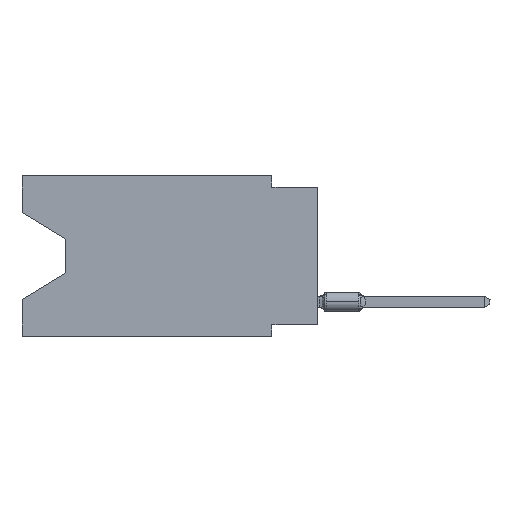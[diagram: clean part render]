
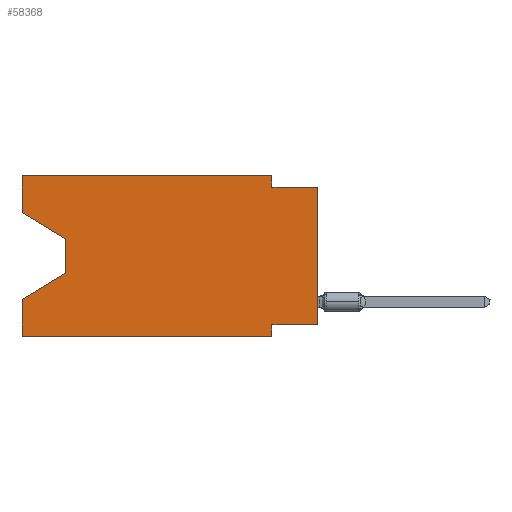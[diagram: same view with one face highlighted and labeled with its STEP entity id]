
A CAD part, left-side view. The second image highlights one B-rep face of the part: STEP entity #58368.
In plain terms, the highlighted planar face has unit normal (-1, 0, 0).
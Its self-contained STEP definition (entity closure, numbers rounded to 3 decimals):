
#1597 = DIRECTION ( 'NONE',  ( 0., -1., 0. ) ) ;
#2646 = CARTESIAN_POINT ( 'NONE',  ( 0., 16.383, -2.038 ) ) ;
#3016 = LINE ( 'NONE', #53191, #84202 ) ;
#3554 = LINE ( 'NONE', #24360, #45992 ) ;
#4073 = LINE ( 'NONE', #61832, #77702 ) ;
#5018 = DIRECTION ( 'NONE',  ( 0., 0., -1. ) ) ;
#6197 = VECTOR ( 'NONE', #53767, 1000. ) ;
#7446 = EDGE_CURVE ( 'NONE', #9179, #8577, #59473, .T. ) ;
#8342 = CARTESIAN_POINT ( 'NONE',  ( 0., 2.54, 0. ) ) ;
#8478 = CARTESIAN_POINT ( 'NONE',  ( 0., 16.383, 0. ) ) ;
#8577 = VERTEX_POINT ( 'NONE', #38698 ) ;
#9179 = VERTEX_POINT ( 'NONE', #23064 ) ;
#10538 = CARTESIAN_POINT ( 'NONE',  ( 0., 16.383, -6.852 ) ) ;
#14163 = ORIENTED_EDGE ( 'NONE', *, *, #7446, .F. ) ;
#16252 = CARTESIAN_POINT ( 'NONE',  ( 0., 0., -0.635 ) ) ;
#16510 = LINE ( 'NONE', #33056, #33289 ) ;
#17475 = CARTESIAN_POINT ( 'NONE',  ( 0., 13.97, -3.505 ) ) ;
#18274 = CARTESIAN_POINT ( 'NONE',  ( 0., 2.54, -8.89 ) ) ;
#18910 = ORIENTED_EDGE ( 'NONE', *, *, #53152, .F. ) ;
#22202 = LINE ( 'NONE', #8478, #68159 ) ;
#22275 = VERTEX_POINT ( 'NONE', #86862 ) ;
#23064 = CARTESIAN_POINT ( 'NONE',  ( 0., 2.54, 0. ) ) ;
#23119 = VERTEX_POINT ( 'NONE', #49735 ) ;
#23192 = CARTESIAN_POINT ( 'NONE',  ( 0., 16.383, 0. ) ) ;
#24360 = CARTESIAN_POINT ( 'NONE',  ( 0., 16.383, -8.89 ) ) ;
#24616 = ORIENTED_EDGE ( 'NONE', *, *, #71028, .T. ) ;
#26470 = EDGE_CURVE ( 'NONE', #22275, #47350, #39522, .T. ) ;
#27247 = LINE ( 'NONE', #18274, #87686 ) ;
#27259 = DIRECTION ( 'NONE',  ( 0., 0., 1. ) ) ;
#27795 = ORIENTED_EDGE ( 'NONE', *, *, #49248, .T. ) ;
#29065 = AXIS2_PLACEMENT_3D ( 'NONE', #48102, #54296, #53832 ) ;
#30268 = DIRECTION ( 'NONE',  ( 0., 0., 1. ) ) ;
#31049 = VECTOR ( 'NONE', #37221, 1000. ) ;
#31284 = VECTOR ( 'NONE', #34938, 1000. ) ;
#33056 = CARTESIAN_POINT ( 'NONE',  ( 0., 0., -8.255 ) ) ;
#33289 = VECTOR ( 'NONE', #83257, 1000. ) ;
#34938 = DIRECTION ( 'NONE',  ( 0., 0., -1. ) ) ;
#35866 = LINE ( 'NONE', #63342, #31284 ) ;
#37221 = DIRECTION ( 'NONE',  ( 0., 0., -1. ) ) ;
#38698 = CARTESIAN_POINT ( 'NONE',  ( 0., 2.54, -0.635 ) ) ;
#39522 = LINE ( 'NONE', #89206, #59727 ) ;
#42939 = VERTEX_POINT ( 'NONE', #63623 ) ;
#43797 = EDGE_CURVE ( 'NONE', #84030, #50709, #67022, .T. ) ;
#43973 = ORIENTED_EDGE ( 'NONE', *, *, #76779, .F. ) ;
#44457 = ORIENTED_EDGE ( 'NONE', *, *, #43797, .T. ) ;
#45992 = VECTOR ( 'NONE', #53250, 1000. ) ;
#47350 = VERTEX_POINT ( 'NONE', #10538 ) ;
#47457 = CARTESIAN_POINT ( 'NONE',  ( 0., 2.54, -8.255 ) ) ;
#48102 = CARTESIAN_POINT ( 'NONE',  ( 0., 16.383, 0. ) ) ;
#48496 = ORIENTED_EDGE ( 'NONE', *, *, #26470, .T. ) ;
#48751 = ORIENTED_EDGE ( 'NONE', *, *, #84985, .F. ) ;
#49248 = EDGE_CURVE ( 'NONE', #23119, #42939, #3554, .T. ) ;
#49735 = CARTESIAN_POINT ( 'NONE',  ( 0., 16.383, -8.89 ) ) ;
#50709 = VERTEX_POINT ( 'NONE', #17475 ) ;
#52830 = ORIENTED_EDGE ( 'NONE', *, *, #90267, .F. ) ;
#53152 = EDGE_CURVE ( 'NONE', #23119, #47350, #88065, .T. ) ;
#53191 = CARTESIAN_POINT ( 'NONE',  ( 0., 0., -0.635 ) ) ;
#53238 = DIRECTION ( 'NONE',  ( 0., 0.855, -0.519 ) ) ;
#53250 = DIRECTION ( 'NONE',  ( 0., -1., 0. ) ) ;
#53767 = DIRECTION ( 'NONE',  ( 0., -0.855, -0.519 ) ) ;
#53832 = DIRECTION ( 'NONE',  ( 0., 0., -1. ) ) ;
#54296 = DIRECTION ( 'NONE',  ( 1., 0., 0. ) ) ;
#58368 = ADVANCED_FACE ( 'NONE', ( #68028 ), #61852, .F. ) ;
#59473 = LINE ( 'NONE', #8342, #31049 ) ;
#59727 = VECTOR ( 'NONE', #53238, 1000. ) ;
#61832 = CARTESIAN_POINT ( 'NONE',  ( 0., 16.383, 0. ) ) ;
#61852 = PLANE ( 'NONE',  #29065 ) ;
#63342 = CARTESIAN_POINT ( 'NONE',  ( 0., 13.97, -3.505 ) ) ;
#63623 = CARTESIAN_POINT ( 'NONE',  ( 0., 2.54, -8.89 ) ) ;
#64370 = EDGE_CURVE ( 'NONE', #70441, #74859, #16510, .T. ) ;
#67022 = LINE ( 'NONE', #2646, #6197 ) ;
#67643 = EDGE_LOOP ( 'NONE', ( #44457, #24616, #48496, #18910, #27795, #52830, #90564, #90434, #48751, #14163, #91104, #43973 ) ) ;
#67654 = EDGE_CURVE ( 'NONE', #82301, #9179, #4073, .T. ) ;
#68028 = FACE_OUTER_BOUND ( 'NONE', #67643, .T. ) ;
#68159 = VECTOR ( 'NONE', #30268, 1000. ) ;
#68173 = VECTOR ( 'NONE', #27259, 1000. ) ;
#70441 = VERTEX_POINT ( 'NONE', #84290 ) ;
#70815 = CARTESIAN_POINT ( 'NONE',  ( 0., 0., 0. ) ) ;
#71028 = EDGE_CURVE ( 'NONE', #50709, #22275, #35866, .T. ) ;
#73861 = DIRECTION ( 'NONE',  ( 0., 0., 1. ) ) ;
#74859 = VERTEX_POINT ( 'NONE', #47457 ) ;
#76050 = LINE ( 'NONE', #70815, #68173 ) ;
#76779 = EDGE_CURVE ( 'NONE', #84030, #82301, #22202, .T. ) ;
#77702 = VECTOR ( 'NONE', #91162, 1000. ) ;
#80689 = VERTEX_POINT ( 'NONE', #16252 ) ;
#82301 = VERTEX_POINT ( 'NONE', #90619 ) ;
#83257 = DIRECTION ( 'NONE',  ( 0., 1., 0. ) ) ;
#84030 = VERTEX_POINT ( 'NONE', #92366 ) ;
#84202 = VECTOR ( 'NONE', #1597, 1000. ) ;
#84290 = CARTESIAN_POINT ( 'NONE',  ( 0., 0., -8.255 ) ) ;
#84985 = EDGE_CURVE ( 'NONE', #8577, #80689, #3016, .T. ) ;
#86862 = CARTESIAN_POINT ( 'NONE',  ( 0., 13.97, -5.385 ) ) ;
#87686 = VECTOR ( 'NONE', #5018, 1000. ) ;
#88065 = LINE ( 'NONE', #23192, #90583 ) ;
#89206 = CARTESIAN_POINT ( 'NONE',  ( 0., 13.97, -5.385 ) ) ;
#90267 = EDGE_CURVE ( 'NONE', #74859, #42939, #27247, .T. ) ;
#90434 = ORIENTED_EDGE ( 'NONE', *, *, #91460, .T. ) ;
#90564 = ORIENTED_EDGE ( 'NONE', *, *, #64370, .F. ) ;
#90583 = VECTOR ( 'NONE', #73861, 1000. ) ;
#90619 = CARTESIAN_POINT ( 'NONE',  ( 0., 16.383, 0. ) ) ;
#91104 = ORIENTED_EDGE ( 'NONE', *, *, #67654, .F. ) ;
#91162 = DIRECTION ( 'NONE',  ( 0., -1., 0. ) ) ;
#91460 = EDGE_CURVE ( 'NONE', #70441, #80689, #76050, .T. ) ;
#92366 = CARTESIAN_POINT ( 'NONE',  ( 0., 16.383, -2.038 ) ) ;
